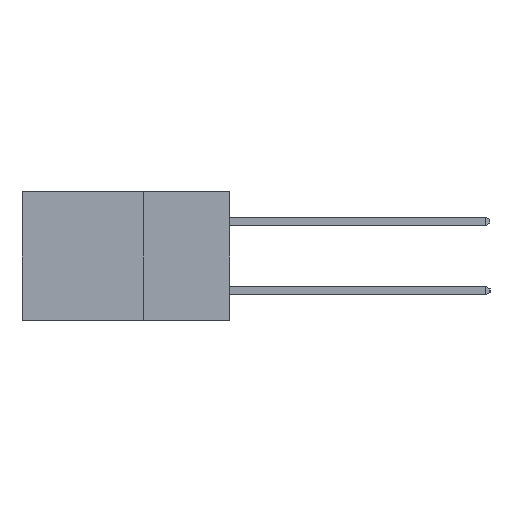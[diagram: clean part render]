
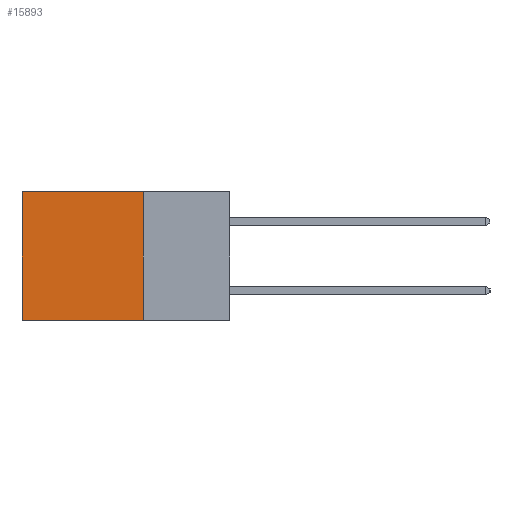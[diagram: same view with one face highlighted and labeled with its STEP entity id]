
A CAD part, left-side view. The second image highlights one B-rep face of the part: STEP entity #15893.
In plain terms, the highlighted planar face has unit normal (-1, 0, 0).
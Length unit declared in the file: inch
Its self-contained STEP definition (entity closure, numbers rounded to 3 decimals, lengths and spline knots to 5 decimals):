
#228 = EDGE_CURVE ( 'NONE', #16880, #13727, #5966, .T. ) ;
#434 = CARTESIAN_POINT ( 'NONE',  ( 0.2615, 0.25, 0. ) ) ;
#1510 = EDGE_CURVE ( 'NONE', #9650, #6110, #13034, .T. ) ;
#1719 = CARTESIAN_POINT ( 'NONE',  ( 0.2615, 0.25, -0.37 ) ) ;
#1727 = AXIS2_PLACEMENT_3D ( 'NONE', #14591, #17229, #9197 ) ;
#3453 = PLANE ( 'NONE',  #1727 ) ;
#4122 = EDGE_CURVE ( 'NONE', #13727, #6110, #14002, .T. ) ;
#4171 = CARTESIAN_POINT ( 'NONE',  ( 0.2615, 0.6, -0.37 ) ) ;
#5005 = CARTESIAN_POINT ( 'NONE',  ( 0.2615, 0.6, -0.37 ) ) ;
#5347 = DIRECTION ( 'NONE',  ( 0., 1., 0. ) ) ;
#5498 = EDGE_CURVE ( 'NONE', #16880, #9650, #16831, .T. ) ;
#5966 = LINE ( 'NONE', #9826, #16363 ) ;
#6041 = ORIENTED_EDGE ( 'NONE', *, *, #1510, .T. ) ;
#6050 = CARTESIAN_POINT ( 'NONE',  ( 0.2615, 0.25, -0.37 ) ) ;
#6110 = VERTEX_POINT ( 'NONE', #5005 ) ;
#6313 = DIRECTION ( 'NONE',  ( 0., 1., 0. ) ) ;
#6498 = CARTESIAN_POINT ( 'NONE',  ( 0.2615, 0.25, 0. ) ) ;
#9197 = DIRECTION ( 'NONE',  ( 0., 0., -1. ) ) ;
#9548 = DIRECTION ( 'NONE',  ( 0., 0., -1. ) ) ;
#9650 = VERTEX_POINT ( 'NONE', #18291 ) ;
#9826 = CARTESIAN_POINT ( 'NONE',  ( 0.2615, 0.25, -0.37 ) ) ;
#10407 = VECTOR ( 'NONE', #5347, 39.37008 ) ;
#10763 = ORIENTED_EDGE ( 'NONE', *, *, #4122, .F. ) ;
#11315 = ORIENTED_EDGE ( 'NONE', *, *, #228, .F. ) ;
#12575 = FACE_OUTER_BOUND ( 'NONE', #13925, .T. ) ;
#13034 = LINE ( 'NONE', #4171, #16548 ) ;
#13319 = VECTOR ( 'NONE', #6313, 39.37008 ) ;
#13727 = VERTEX_POINT ( 'NONE', #1719 ) ;
#13925 = EDGE_LOOP ( 'NONE', ( #6041, #10763, #11315, #17697 ) ) ;
#14002 = LINE ( 'NONE', #6050, #10407 ) ;
#14591 = CARTESIAN_POINT ( 'NONE',  ( 0.2615, 0.25, -0.37 ) ) ;
#15893 = ADVANCED_FACE ( 'NONE', ( #12575 ), #3453, .F. ) ;
#16363 = VECTOR ( 'NONE', #9548, 39.37008 ) ;
#16388 = DIRECTION ( 'NONE',  ( 0., 0., -1. ) ) ;
#16548 = VECTOR ( 'NONE', #16388, 39.37008 ) ;
#16831 = LINE ( 'NONE', #6498, #13319 ) ;
#16880 = VERTEX_POINT ( 'NONE', #434 ) ;
#17229 = DIRECTION ( 'NONE',  ( 1., 0., 0. ) ) ;
#17697 = ORIENTED_EDGE ( 'NONE', *, *, #5498, .T. ) ;
#18291 = CARTESIAN_POINT ( 'NONE',  ( 0.2615, 0.6, 0. ) ) ;
